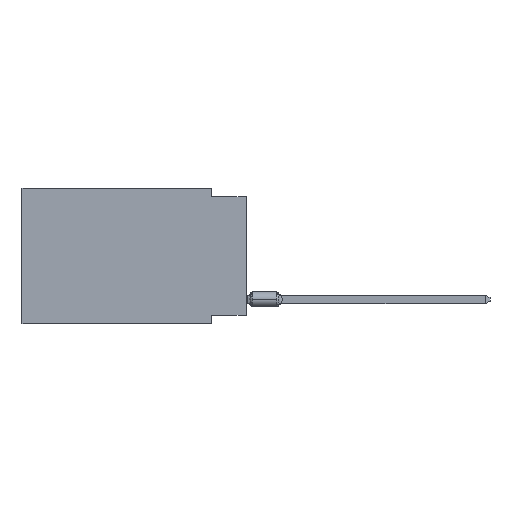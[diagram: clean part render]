
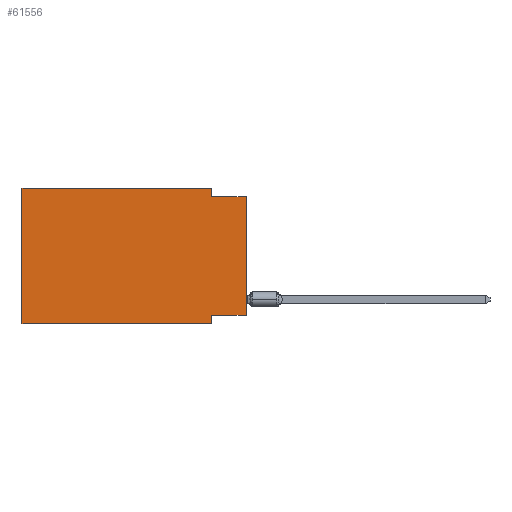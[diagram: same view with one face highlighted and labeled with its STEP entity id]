
A CAD part, left-side view. The second image highlights one B-rep face of the part: STEP entity #61556.
In plain terms, the highlighted planar face has unit normal (-1, 0, 0).
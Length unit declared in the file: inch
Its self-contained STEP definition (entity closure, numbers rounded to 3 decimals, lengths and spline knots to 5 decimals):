
#2069 = VECTOR ( 'NONE', #57265, 39.37008 ) ;
#3012 = DIRECTION ( 'NONE',  ( 0., -1., 0. ) ) ;
#3105 = LINE ( 'NONE', #25243, #57639 ) ;
#3487 = AXIS2_PLACEMENT_3D ( 'NONE', #41846, #63235, #23735 ) ;
#6140 = VERTEX_POINT ( 'NONE', #17402 ) ;
#6154 = EDGE_CURVE ( 'NONE', #55036, #24592, #46745, .T. ) ;
#8253 = ORIENTED_EDGE ( 'NONE', *, *, #66486, .T. ) ;
#8851 = DIRECTION ( 'NONE',  ( 0., 0., -1. ) ) ;
#11182 = CARTESIAN_POINT ( 'NONE',  ( 0., 0.645, -0.39 ) ) ;
#13562 = PLANE ( 'NONE',  #3487 ) ;
#13925 = VERTEX_POINT ( 'NONE', #15688 ) ;
#13992 = LINE ( 'NONE', #31030, #39678 ) ;
#15640 = CARTESIAN_POINT ( 'NONE',  ( 0., 0., -0.365 ) ) ;
#15688 = CARTESIAN_POINT ( 'NONE',  ( 0., 0.645, 0. ) ) ;
#17402 = CARTESIAN_POINT ( 'NONE',  ( 0., 0.1, -0.365 ) ) ;
#18205 = VECTOR ( 'NONE', #8851, 39.37008 ) ;
#19325 = VECTOR ( 'NONE', #3012, 39.37008 ) ;
#19795 = DIRECTION ( 'NONE',  ( 0., 0., 1. ) ) ;
#23735 = DIRECTION ( 'NONE',  ( 0., 0., -1. ) ) ;
#24466 = LINE ( 'NONE', #59255, #18205 ) ;
#24592 = VERTEX_POINT ( 'NONE', #51301 ) ;
#24625 = CARTESIAN_POINT ( 'NONE',  ( 0., 0., 0. ) ) ;
#25243 = CARTESIAN_POINT ( 'NONE',  ( 0., 0.645, 0. ) ) ;
#26786 = EDGE_CURVE ( 'NONE', #68699, #48069, #46327, .T. ) ;
#27268 = EDGE_CURVE ( 'NONE', #6140, #30798, #24466, .T. ) ;
#28864 = ORIENTED_EDGE ( 'NONE', *, *, #34812, .F. ) ;
#29538 = VECTOR ( 'NONE', #71358, 39.37008 ) ;
#30798 = VERTEX_POINT ( 'NONE', #39510 ) ;
#31030 = CARTESIAN_POINT ( 'NONE',  ( 0., 0., -0.365 ) ) ;
#31344 = CARTESIAN_POINT ( 'NONE',  ( 0., 0.645, 0. ) ) ;
#34127 = ORIENTED_EDGE ( 'NONE', *, *, #41084, .F. ) ;
#34610 = LINE ( 'NONE', #41466, #19325 ) ;
#34812 = EDGE_CURVE ( 'NONE', #55036, #6140, #13992, .T. ) ;
#39185 = VECTOR ( 'NONE', #51059, 39.37008 ) ;
#39510 = CARTESIAN_POINT ( 'NONE',  ( 0., 0.1, -0.39 ) ) ;
#39678 = VECTOR ( 'NONE', #41558, 39.37008 ) ;
#40380 = ORIENTED_EDGE ( 'NONE', *, *, #26786, .F. ) ;
#40422 = FACE_OUTER_BOUND ( 'NONE', #40466, .T. ) ;
#40466 = EDGE_LOOP ( 'NONE', ( #43418, #34127, #40380, #57341, #60796, #8253, #45473, #28864 ) ) ;
#41084 = EDGE_CURVE ( 'NONE', #48069, #24592, #34610, .T. ) ;
#41466 = CARTESIAN_POINT ( 'NONE',  ( 0., 0., -0.025 ) ) ;
#41558 = DIRECTION ( 'NONE',  ( 0., 1., 0. ) ) ;
#41846 = CARTESIAN_POINT ( 'NONE',  ( 0., 0.645, 0. ) ) ;
#43418 = ORIENTED_EDGE ( 'NONE', *, *, #6154, .T. ) ;
#44091 = EDGE_CURVE ( 'NONE', #48693, #13925, #3105, .T. ) ;
#45473 = ORIENTED_EDGE ( 'NONE', *, *, #27268, .F. ) ;
#46327 = LINE ( 'NONE', #68422, #39185 ) ;
#46745 = LINE ( 'NONE', #24625, #2069 ) ;
#47310 = LINE ( 'NONE', #31344, #66659 ) ;
#48023 = DIRECTION ( 'NONE',  ( 0., -1., 0. ) ) ;
#48069 = VERTEX_POINT ( 'NONE', #67832 ) ;
#48693 = VERTEX_POINT ( 'NONE', #60366 ) ;
#51059 = DIRECTION ( 'NONE',  ( 0., 0., -1. ) ) ;
#51301 = CARTESIAN_POINT ( 'NONE',  ( 0., 0., -0.025 ) ) ;
#51377 = CARTESIAN_POINT ( 'NONE',  ( 0., 0.1, 0. ) ) ;
#55036 = VERTEX_POINT ( 'NONE', #15640 ) ;
#57265 = DIRECTION ( 'NONE',  ( 0., 0., 1. ) ) ;
#57341 = ORIENTED_EDGE ( 'NONE', *, *, #67140, .F. ) ;
#57639 = VECTOR ( 'NONE', #19795, 39.37008 ) ;
#59255 = CARTESIAN_POINT ( 'NONE',  ( 0., 0.1, -0.39 ) ) ;
#60366 = CARTESIAN_POINT ( 'NONE',  ( 0., 0.645, -0.39 ) ) ;
#60796 = ORIENTED_EDGE ( 'NONE', *, *, #44091, .F. ) ;
#60861 = LINE ( 'NONE', #11182, #29538 ) ;
#61556 = ADVANCED_FACE ( 'NONE', ( #40422 ), #13562, .F. ) ;
#63235 = DIRECTION ( 'NONE',  ( 1., 0., 0. ) ) ;
#66486 = EDGE_CURVE ( 'NONE', #48693, #30798, #60861, .T. ) ;
#66659 = VECTOR ( 'NONE', #48023, 39.37008 ) ;
#67140 = EDGE_CURVE ( 'NONE', #13925, #68699, #47310, .T. ) ;
#67832 = CARTESIAN_POINT ( 'NONE',  ( 0., 0.1, -0.025 ) ) ;
#68422 = CARTESIAN_POINT ( 'NONE',  ( 0., 0.1, 0. ) ) ;
#68699 = VERTEX_POINT ( 'NONE', #51377 ) ;
#71358 = DIRECTION ( 'NONE',  ( 0., -1., 0. ) ) ;
